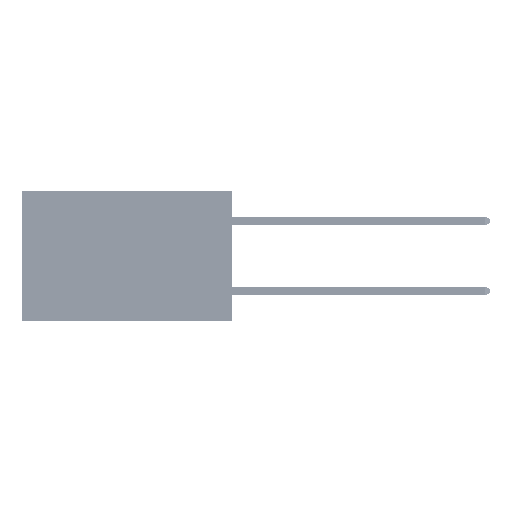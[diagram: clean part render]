
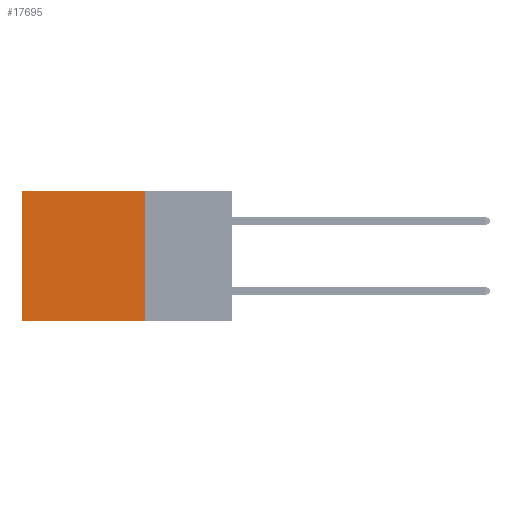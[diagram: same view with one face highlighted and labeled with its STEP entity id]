
A CAD part, left-side view. The second image highlights one B-rep face of the part: STEP entity #17695.
In plain terms, the highlighted planar face has unit normal (-1, 0, 0).
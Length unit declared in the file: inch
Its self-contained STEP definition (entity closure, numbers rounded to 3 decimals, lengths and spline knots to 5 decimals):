
#115 = VERTEX_POINT ( 'NONE', #1871 ) ;
#334 = EDGE_CURVE ( 'NONE', #115, #9794, #33270, .T. ) ;
#1871 = CARTESIAN_POINT ( 'NONE',  ( 0.2875, 0.25, -0.37 ) ) ;
#1982 = VERTEX_POINT ( 'NONE', #8246 ) ;
#2020 = ORIENTED_EDGE ( 'NONE', *, *, #334, .F. ) ;
#4758 = ORIENTED_EDGE ( 'NONE', *, *, #41495, .F. ) ;
#5847 = VERTEX_POINT ( 'NONE', #17568 ) ;
#6914 = ORIENTED_EDGE ( 'NONE', *, *, #17122, .T. ) ;
#7082 = CARTESIAN_POINT ( 'NONE',  ( 0.2875, 0.25, 0. ) ) ;
#8005 = VECTOR ( 'NONE', #43894, 39.37008 ) ;
#8246 = CARTESIAN_POINT ( 'NONE',  ( 0.2875, 0.25, 0. ) ) ;
#9794 = VERTEX_POINT ( 'NONE', #38923 ) ;
#9861 = LINE ( 'NONE', #40021, #39526 ) ;
#10107 = DIRECTION ( 'NONE',  ( 0., 1., 0. ) ) ;
#10696 = FACE_OUTER_BOUND ( 'NONE', #29819, .T. ) ;
#14070 = VECTOR ( 'NONE', #39565, 39.37008 ) ;
#17122 = EDGE_CURVE ( 'NONE', #1982, #5847, #9861, .T. ) ;
#17568 = CARTESIAN_POINT ( 'NONE',  ( 0.2875, 0.6, 0. ) ) ;
#17695 = ADVANCED_FACE ( 'NONE', ( #10696 ), #40153, .F. ) ;
#18070 = LINE ( 'NONE', #46354, #14070 ) ;
#21813 = DIRECTION ( 'NONE',  ( 1., 0., 0. ) ) ;
#22163 = ORIENTED_EDGE ( 'NONE', *, *, #44406, .T. ) ;
#26612 = DIRECTION ( 'NONE',  ( 0., 0., -1. ) ) ;
#29819 = EDGE_LOOP ( 'NONE', ( #22163, #2020, #4758, #6914 ) ) ;
#33270 = LINE ( 'NONE', #40497, #8005 ) ;
#33988 = CARTESIAN_POINT ( 'NONE',  ( 0.2875, 0.25, 0. ) ) ;
#38923 = CARTESIAN_POINT ( 'NONE',  ( 0.2875, 0.6, -0.37 ) ) ;
#39526 = VECTOR ( 'NONE', #10107, 39.37008 ) ;
#39565 = DIRECTION ( 'NONE',  ( 0., 0., -1. ) ) ;
#40021 = CARTESIAN_POINT ( 'NONE',  ( 0.2875, 0.25, 0. ) ) ;
#40153 = PLANE ( 'NONE',  #46536 ) ;
#40497 = CARTESIAN_POINT ( 'NONE',  ( 0.2875, 0.25, -0.37 ) ) ;
#41003 = DIRECTION ( 'NONE',  ( 0., 0., -1. ) ) ;
#41495 = EDGE_CURVE ( 'NONE', #1982, #115, #44160, .T. ) ;
#43894 = DIRECTION ( 'NONE',  ( 0., 1., 0. ) ) ;
#44160 = LINE ( 'NONE', #33988, #47176 ) ;
#44406 = EDGE_CURVE ( 'NONE', #5847, #9794, #18070, .T. ) ;
#46354 = CARTESIAN_POINT ( 'NONE',  ( 0.2875, 0.6, 0. ) ) ;
#46536 = AXIS2_PLACEMENT_3D ( 'NONE', #7082, #21813, #26612 ) ;
#47176 = VECTOR ( 'NONE', #41003, 39.37008 ) ;
